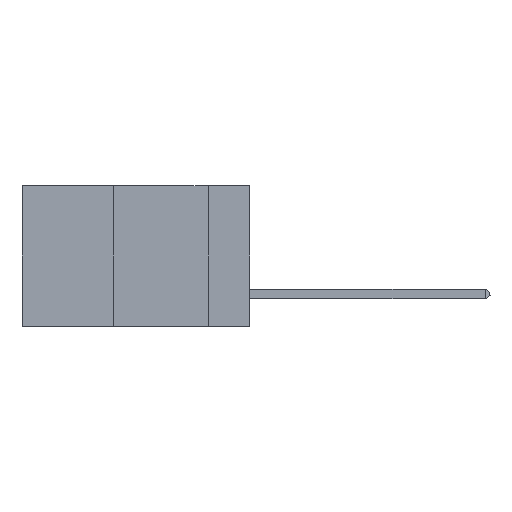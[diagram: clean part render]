
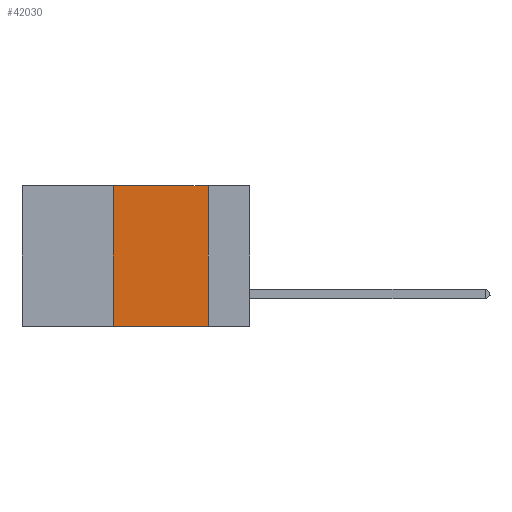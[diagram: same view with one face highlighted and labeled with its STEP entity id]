
A CAD part, left-side view. The second image highlights one B-rep face of the part: STEP entity #42030.
In plain terms, the highlighted planar face has unit normal (-1, 0, 0).
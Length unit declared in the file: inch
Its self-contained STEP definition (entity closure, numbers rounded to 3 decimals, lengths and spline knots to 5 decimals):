
#1862 = ORIENTED_EDGE ( 'NONE', *, *, #14328, .F. ) ;
#5410 = VECTOR ( 'NONE', #24575, 39.37008 ) ;
#5840 = CARTESIAN_POINT ( 'NONE',  ( 0., 0.36, -0.37 ) ) ;
#6318 = DIRECTION ( 'NONE',  ( 0., 0., -1. ) ) ;
#9164 = LINE ( 'NONE', #44382, #28374 ) ;
#11977 = VECTOR ( 'NONE', #30034, 39.37008 ) ;
#12259 = LINE ( 'NONE', #37651, #19365 ) ;
#14328 = EDGE_CURVE ( 'NONE', #25159, #40171, #20186, .T. ) ;
#16746 = FACE_OUTER_BOUND ( 'NONE', #28958, .T. ) ;
#16964 = DIRECTION ( 'NONE',  ( 0., -1., 0. ) ) ;
#17729 = EDGE_CURVE ( 'NONE', #25159, #28253, #12259, .T. ) ;
#18478 = EDGE_CURVE ( 'NONE', #40171, #32190, #22347, .T. ) ;
#19365 = VECTOR ( 'NONE', #16964, 39.37008 ) ;
#19895 = CARTESIAN_POINT ( 'NONE',  ( 0., 0.36, 0. ) ) ;
#20186 = LINE ( 'NONE', #19895, #11977 ) ;
#21048 = ORIENTED_EDGE ( 'NONE', *, *, #33304, .F. ) ;
#22347 = LINE ( 'NONE', #38658, #5410 ) ;
#24575 = DIRECTION ( 'NONE',  ( 0., -1., 0. ) ) ;
#24698 = CARTESIAN_POINT ( 'NONE',  ( 0., 0.11, -0.37 ) ) ;
#25159 = VERTEX_POINT ( 'NONE', #5840 ) ;
#27291 = CARTESIAN_POINT ( 'NONE',  ( 0., 0.6, 0. ) ) ;
#28253 = VERTEX_POINT ( 'NONE', #24698 ) ;
#28374 = VECTOR ( 'NONE', #44239, 39.37008 ) ;
#28958 = EDGE_LOOP ( 'NONE', ( #21048, #44639, #1862, #36438 ) ) ;
#30034 = DIRECTION ( 'NONE',  ( 0., 0., 1. ) ) ;
#31265 = PLANE ( 'NONE',  #42950 ) ;
#32190 = VERTEX_POINT ( 'NONE', #37907 ) ;
#33304 = EDGE_CURVE ( 'NONE', #32190, #28253, #9164, .T. ) ;
#36167 = CARTESIAN_POINT ( 'NONE',  ( 0., 0.36, 0. ) ) ;
#36438 = ORIENTED_EDGE ( 'NONE', *, *, #17729, .T. ) ;
#37651 = CARTESIAN_POINT ( 'NONE',  ( 0., 0.6, -0.37 ) ) ;
#37907 = CARTESIAN_POINT ( 'NONE',  ( 0., 0.11, 0. ) ) ;
#38658 = CARTESIAN_POINT ( 'NONE',  ( 0., 0.6, 0. ) ) ;
#40171 = VERTEX_POINT ( 'NONE', #36167 ) ;
#41357 = DIRECTION ( 'NONE',  ( 1., 0., 0. ) ) ;
#42030 = ADVANCED_FACE ( 'NONE', ( #16746 ), #31265, .F. ) ;
#42950 = AXIS2_PLACEMENT_3D ( 'NONE', #27291, #41357, #6318 ) ;
#44239 = DIRECTION ( 'NONE',  ( 0., 0., -1. ) ) ;
#44382 = CARTESIAN_POINT ( 'NONE',  ( 0., 0.11, 0. ) ) ;
#44639 = ORIENTED_EDGE ( 'NONE', *, *, #18478, .F. ) ;
